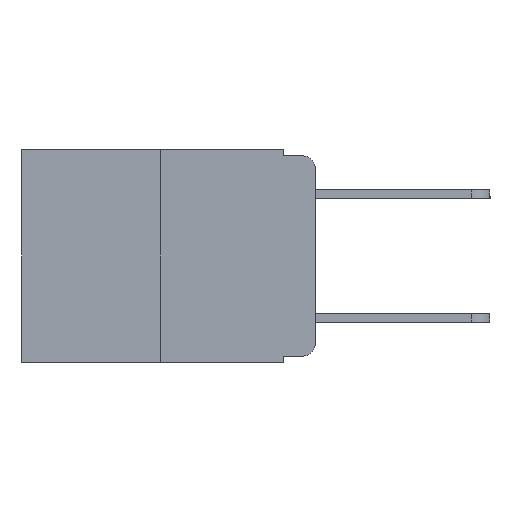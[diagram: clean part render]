
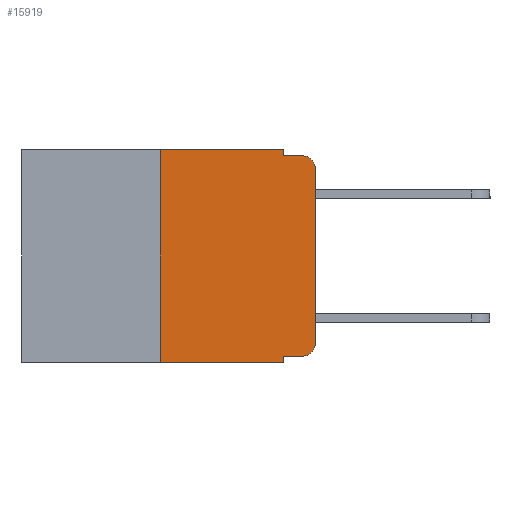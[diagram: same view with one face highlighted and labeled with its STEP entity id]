
A CAD part, left-side view. The second image highlights one B-rep face of the part: STEP entity #15919.
In plain terms, the highlighted planar face has unit normal (-1, 0, 0).
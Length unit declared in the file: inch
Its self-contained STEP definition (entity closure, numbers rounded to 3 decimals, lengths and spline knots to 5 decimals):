
#56 = EDGE_CURVE ( 'NONE', #10282, #9176, #22918, .T. ) ;
#386 = ORIENTED_EDGE ( 'NONE', *, *, #5477, .T. ) ;
#876 = PLANE ( 'NONE',  #22929 ) ;
#912 = VECTOR ( 'NONE', #15959, 39.37008 ) ;
#1280 = VERTEX_POINT ( 'NONE', #16374 ) ;
#1841 = VERTEX_POINT ( 'NONE', #5035 ) ;
#2232 = CARTESIAN_POINT ( 'NONE',  ( 0., 0., -0.313 ) ) ;
#2322 = CARTESIAN_POINT ( 'NONE',  ( 0., 0.25, -0.343 ) ) ;
#2489 = ORIENTED_EDGE ( 'NONE', *, *, #19028, .F. ) ;
#2972 = DIRECTION ( 'NONE',  ( 0., -1., 0. ) ) ;
#3058 = VECTOR ( 'NONE', #2972, 39.37008 ) ;
#3085 = CARTESIAN_POINT ( 'NONE',  ( 0., 0.051, 0. ) ) ;
#3283 = VECTOR ( 'NONE', #18059, 39.37008 ) ;
#3426 = CARTESIAN_POINT ( 'NONE',  ( 0., 0.051, 0. ) ) ;
#3579 = CIRCLE ( 'NONE', #20398, 0.02 ) ;
#3655 = LINE ( 'NONE', #17650, #3058 ) ;
#3792 = VERTEX_POINT ( 'NONE', #9977 ) ;
#4017 = CARTESIAN_POINT ( 'NONE',  ( 0., 0.25, 0. ) ) ;
#4331 = CARTESIAN_POINT ( 'NONE',  ( 0., 0.02, -0.03 ) ) ;
#4994 = VERTEX_POINT ( 'NONE', #4017 ) ;
#5015 = VECTOR ( 'NONE', #21993, 39.37008 ) ;
#5035 = CARTESIAN_POINT ( 'NONE',  ( 0., 0.02, -0.333 ) ) ;
#5386 = DIRECTION ( 'NONE',  ( 0., 0., -1. ) ) ;
#5420 = VERTEX_POINT ( 'NONE', #8922 ) ;
#5436 = ORIENTED_EDGE ( 'NONE', *, *, #16650, .F. ) ;
#5477 = EDGE_CURVE ( 'NONE', #23119, #5480, #12632, .T. ) ;
#5480 = VERTEX_POINT ( 'NONE', #10868 ) ;
#6000 = ORIENTED_EDGE ( 'NONE', *, *, #15449, .T. ) ;
#6189 = DIRECTION ( 'NONE',  ( 0., 0., -1. ) ) ;
#6287 = ORIENTED_EDGE ( 'NONE', *, *, #22522, .T. ) ;
#6554 = CARTESIAN_POINT ( 'NONE',  ( 0., 0.473, 0. ) ) ;
#7462 = VERTEX_POINT ( 'NONE', #18291 ) ;
#7837 = DIRECTION ( 'NONE',  ( 0., 0., 1. ) ) ;
#7944 = CARTESIAN_POINT ( 'NONE',  ( 0., 0., 0. ) ) ;
#8653 = ORIENTED_EDGE ( 'NONE', *, *, #15214, .F. ) ;
#8922 = CARTESIAN_POINT ( 'NONE',  ( 0., 0.02, -0.01 ) ) ;
#8954 = LINE ( 'NONE', #15243, #17980 ) ;
#9096 = CARTESIAN_POINT ( 'NONE',  ( 0., 0.02, -0.313 ) ) ;
#9176 = VERTEX_POINT ( 'NONE', #17231 ) ;
#9668 = AXIS2_PLACEMENT_3D ( 'NONE', #9096, #21597, #10970 ) ;
#9977 = CARTESIAN_POINT ( 'NONE',  ( 0., 0.051, -0.01 ) ) ;
#10282 = VERTEX_POINT ( 'NONE', #2232 ) ;
#10351 = DIRECTION ( 'NONE',  ( 0., -1., 0. ) ) ;
#10683 = LINE ( 'NONE', #22753, #15448 ) ;
#10698 = ORIENTED_EDGE ( 'NONE', *, *, #56, .T. ) ;
#10868 = CARTESIAN_POINT ( 'NONE',  ( 0., 0.051, -0.343 ) ) ;
#10970 = DIRECTION ( 'NONE',  ( 0., 0., -1. ) ) ;
#10997 = ORIENTED_EDGE ( 'NONE', *, *, #14295, .T. ) ;
#11407 = CARTESIAN_POINT ( 'NONE',  ( 0., 0.25, 0. ) ) ;
#11587 = EDGE_LOOP ( 'NONE', ( #10698, #6287, #16016, #2489, #8653, #18255, #386, #5436, #6000, #10997 ) ) ;
#12196 = DIRECTION ( 'NONE',  ( 0., 0., -1. ) ) ;
#12241 = VECTOR ( 'NONE', #5386, 39.37008 ) ;
#12632 = LINE ( 'NONE', #16278, #3283 ) ;
#14295 = EDGE_CURVE ( 'NONE', #1841, #10282, #16963, .T. ) ;
#15214 = EDGE_CURVE ( 'NONE', #4994, #1280, #8954, .T. ) ;
#15243 = CARTESIAN_POINT ( 'NONE',  ( 0., 0.473, 0. ) ) ;
#15349 = LINE ( 'NONE', #11407, #5015 ) ;
#15448 = VECTOR ( 'NONE', #10351, 39.37008 ) ;
#15449 = EDGE_CURVE ( 'NONE', #7462, #1841, #3655, .T. ) ;
#15919 = ADVANCED_FACE ( 'NONE', ( #16557 ), #876, .F. ) ;
#15959 = DIRECTION ( 'NONE',  ( 0., 0., -1. ) ) ;
#16016 = ORIENTED_EDGE ( 'NONE', *, *, #21364, .F. ) ;
#16278 = CARTESIAN_POINT ( 'NONE',  ( 0., 0.473, -0.343 ) ) ;
#16374 = CARTESIAN_POINT ( 'NONE',  ( 0., 0.051, 0. ) ) ;
#16557 = FACE_OUTER_BOUND ( 'NONE', #11587, .T. ) ;
#16650 = EDGE_CURVE ( 'NONE', #7462, #5480, #19835, .T. ) ;
#16963 = CIRCLE ( 'NONE', #9668, 0.02 ) ;
#16964 = LINE ( 'NONE', #3426, #12241 ) ;
#17046 = DIRECTION ( 'NONE',  ( 0., -1., 0. ) ) ;
#17135 = DIRECTION ( 'NONE',  ( -1., 0., 0. ) ) ;
#17231 = CARTESIAN_POINT ( 'NONE',  ( 0., 0., -0.03 ) ) ;
#17650 = CARTESIAN_POINT ( 'NONE',  ( 0., 0.051, -0.333 ) ) ;
#17746 = VECTOR ( 'NONE', #7837, 39.37008 ) ;
#17839 = EDGE_CURVE ( 'NONE', #23119, #4994, #15349, .T. ) ;
#17980 = VECTOR ( 'NONE', #17046, 39.37008 ) ;
#18059 = DIRECTION ( 'NONE',  ( 0., -1., 0. ) ) ;
#18255 = ORIENTED_EDGE ( 'NONE', *, *, #17839, .F. ) ;
#18291 = CARTESIAN_POINT ( 'NONE',  ( 0., 0.051, -0.333 ) ) ;
#19028 = EDGE_CURVE ( 'NONE', #1280, #3792, #16964, .T. ) ;
#19835 = LINE ( 'NONE', #3085, #912 ) ;
#20398 = AXIS2_PLACEMENT_3D ( 'NONE', #4331, #17135, #6189 ) ;
#21364 = EDGE_CURVE ( 'NONE', #3792, #5420, #10683, .T. ) ;
#21597 = DIRECTION ( 'NONE',  ( -1., 0., 0. ) ) ;
#21993 = DIRECTION ( 'NONE',  ( 0., 0., 1. ) ) ;
#22522 = EDGE_CURVE ( 'NONE', #9176, #5420, #3579, .T. ) ;
#22739 = DIRECTION ( 'NONE',  ( 1., 0., 0. ) ) ;
#22753 = CARTESIAN_POINT ( 'NONE',  ( 0., 0.051, -0.01 ) ) ;
#22918 = LINE ( 'NONE', #7944, #17746 ) ;
#22929 = AXIS2_PLACEMENT_3D ( 'NONE', #6554, #22739, #12196 ) ;
#23119 = VERTEX_POINT ( 'NONE', #2322 ) ;
